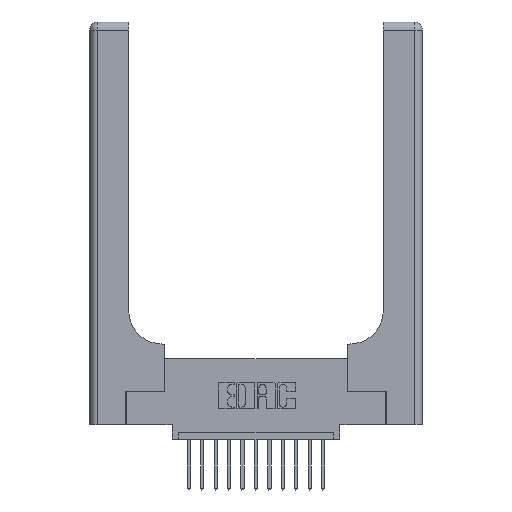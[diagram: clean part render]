
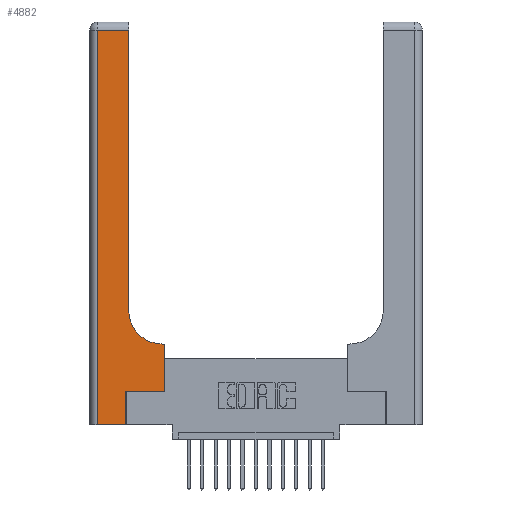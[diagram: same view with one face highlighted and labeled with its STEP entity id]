
A CAD part, top view. The second image highlights one B-rep face of the part: STEP entity #4882.
In plain terms, the highlighted planar face has unit normal (0, 0, 1).
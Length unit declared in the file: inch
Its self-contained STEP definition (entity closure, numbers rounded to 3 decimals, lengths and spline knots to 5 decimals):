
#36 = DIRECTION ( 'NONE',  ( 0., 0., -1. ) ) ;
#276 = DIRECTION ( 'NONE',  ( 1., 0., 0. ) ) ;
#400 = CARTESIAN_POINT ( 'NONE',  ( 0., 0., 0.37 ) ) ;
#878 = ORIENTED_EDGE ( 'NONE', *, *, #15073, .T. ) ;
#969 = VERTEX_POINT ( 'NONE', #14582 ) ;
#1073 = LINE ( 'NONE', #11473, #13526 ) ;
#1223 = VERTEX_POINT ( 'NONE', #12490 ) ;
#1667 = CARTESIAN_POINT ( 'NONE',  ( 0.269, 0.25, 0.37 ) ) ;
#1850 = ORIENTED_EDGE ( 'NONE', *, *, #3347, .T. ) ;
#2121 = CARTESIAN_POINT ( 'NONE',  ( 0., 2.94, 0.37 ) ) ;
#2129 = ORIENTED_EDGE ( 'NONE', *, *, #4717, .T. ) ;
#2861 = ORIENTED_EDGE ( 'NONE', *, *, #14186, .T. ) ;
#2899 = DIRECTION ( 'NONE',  ( 1., 0., 0. ) ) ;
#3139 = AXIS2_PLACEMENT_3D ( 'NONE', #8281, #9759, #2899 ) ;
#3347 = EDGE_CURVE ( 'NONE', #5536, #5917, #17008, .T. ) ;
#3512 = CARTESIAN_POINT ( 'NONE',  ( 0.2915, 0.85, 0.37 ) ) ;
#4115 = CARTESIAN_POINT ( 'NONE',  ( 0., 3., 0.37 ) ) ;
#4123 = EDGE_CURVE ( 'NONE', #16285, #1223, #1073, .T. ) ;
#4235 = LINE ( 'NONE', #8322, #8329 ) ;
#4462 = CARTESIAN_POINT ( 'NONE',  ( 0.5585, 0.6, 0.37 ) ) ;
#4463 = VERTEX_POINT ( 'NONE', #1667 ) ;
#4717 = EDGE_CURVE ( 'NONE', #4463, #969, #16327, .T. ) ;
#4777 = EDGE_LOOP ( 'NONE', ( #10284, #878, #17659, #6571, #2861, #2129, #16688, #1850, #13131 ) ) ;
#4882 = ADVANCED_FACE ( 'NONE', ( #15871 ), #12316, .F. ) ;
#4989 = EDGE_CURVE ( 'NONE', #5087, #7034, #6086, .T. ) ;
#5019 = DIRECTION ( 'NONE',  ( 0., -1., 0. ) ) ;
#5087 = VERTEX_POINT ( 'NONE', #3512 ) ;
#5424 = CARTESIAN_POINT ( 'NONE',  ( 0.06, 2.94, 0.37 ) ) ;
#5536 = VERTEX_POINT ( 'NONE', #4462 ) ;
#5917 = VERTEX_POINT ( 'NONE', #10873 ) ;
#6086 = LINE ( 'NONE', #16816, #13523 ) ;
#6274 = AXIS2_PLACEMENT_3D ( 'NONE', #4115, #36, #13610 ) ;
#6442 = CARTESIAN_POINT ( 'NONE',  ( 0.5585, 0.25, 0.37 ) ) ;
#6536 = EDGE_CURVE ( 'NONE', #969, #5536, #15601, .T. ) ;
#6571 = ORIENTED_EDGE ( 'NONE', *, *, #9074, .T. ) ;
#6749 = CIRCLE ( 'NONE', #3139, 0.25 ) ;
#7034 = VERTEX_POINT ( 'NONE', #16809 ) ;
#7374 = VECTOR ( 'NONE', #9110, 39.37008 ) ;
#7642 = DIRECTION ( 'NONE',  ( 0., 1., 0. ) ) ;
#8281 = CARTESIAN_POINT ( 'NONE',  ( 0.5415, 0.85, 0.37 ) ) ;
#8322 = CARTESIAN_POINT ( 'NONE',  ( 0.269, 0., 0.37 ) ) ;
#8329 = VECTOR ( 'NONE', #16538, 39.37008 ) ;
#8649 = DIRECTION ( 'NONE',  ( 0., 1., 0. ) ) ;
#9071 = CARTESIAN_POINT ( 'NONE',  ( 0.2915, 0.6, 0.37 ) ) ;
#9074 = EDGE_CURVE ( 'NONE', #1223, #13228, #10211, .T. ) ;
#9110 = DIRECTION ( 'NONE',  ( 1., 0., 0. ) ) ;
#9759 = DIRECTION ( 'NONE',  ( 0., 0., -1. ) ) ;
#10211 = LINE ( 'NONE', #400, #13172 ) ;
#10284 = ORIENTED_EDGE ( 'NONE', *, *, #4989, .T. ) ;
#10395 = VECTOR ( 'NONE', #14461, 39.37008 ) ;
#10873 = CARTESIAN_POINT ( 'NONE',  ( 0.5415, 0.6, 0.37 ) ) ;
#11473 = CARTESIAN_POINT ( 'NONE',  ( 0.06, 3., 0.37 ) ) ;
#12316 = PLANE ( 'NONE',  #6274 ) ;
#12490 = CARTESIAN_POINT ( 'NONE',  ( 0.06, 0., 0.37 ) ) ;
#12943 = DIRECTION ( 'NONE',  ( -1., 0., 0. ) ) ;
#13131 = ORIENTED_EDGE ( 'NONE', *, *, #17001, .T. ) ;
#13172 = VECTOR ( 'NONE', #276, 39.37008 ) ;
#13228 = VERTEX_POINT ( 'NONE', #17767 ) ;
#13523 = VECTOR ( 'NONE', #8649, 39.37008 ) ;
#13526 = VECTOR ( 'NONE', #5019, 39.37008 ) ;
#13549 = VECTOR ( 'NONE', #12943, 39.37008 ) ;
#13610 = DIRECTION ( 'NONE',  ( -1., 0., 0. ) ) ;
#14022 = LINE ( 'NONE', #2121, #10395 ) ;
#14186 = EDGE_CURVE ( 'NONE', #13228, #4463, #4235, .T. ) ;
#14461 = DIRECTION ( 'NONE',  ( -1., 0., 0. ) ) ;
#14582 = CARTESIAN_POINT ( 'NONE',  ( 0.5585, 0.25, 0.37 ) ) ;
#15073 = EDGE_CURVE ( 'NONE', #7034, #16285, #14022, .T. ) ;
#15601 = LINE ( 'NONE', #6442, #16050 ) ;
#15871 = FACE_OUTER_BOUND ( 'NONE', #4777, .T. ) ;
#15889 = CARTESIAN_POINT ( 'NONE',  ( 0.269, 0.25, 0.37 ) ) ;
#16050 = VECTOR ( 'NONE', #7642, 39.37008 ) ;
#16285 = VERTEX_POINT ( 'NONE', #5424 ) ;
#16327 = LINE ( 'NONE', #15889, #7374 ) ;
#16538 = DIRECTION ( 'NONE',  ( 0., 1., 0. ) ) ;
#16688 = ORIENTED_EDGE ( 'NONE', *, *, #6536, .T. ) ;
#16809 = CARTESIAN_POINT ( 'NONE',  ( 0.2915, 2.94, 0.37 ) ) ;
#16816 = CARTESIAN_POINT ( 'NONE',  ( 0.2915, 3., 0.37 ) ) ;
#17001 = EDGE_CURVE ( 'NONE', #5917, #5087, #6749, .T. ) ;
#17008 = LINE ( 'NONE', #9071, #13549 ) ;
#17659 = ORIENTED_EDGE ( 'NONE', *, *, #4123, .T. ) ;
#17767 = CARTESIAN_POINT ( 'NONE',  ( 0.269, 0., 0.37 ) ) ;
